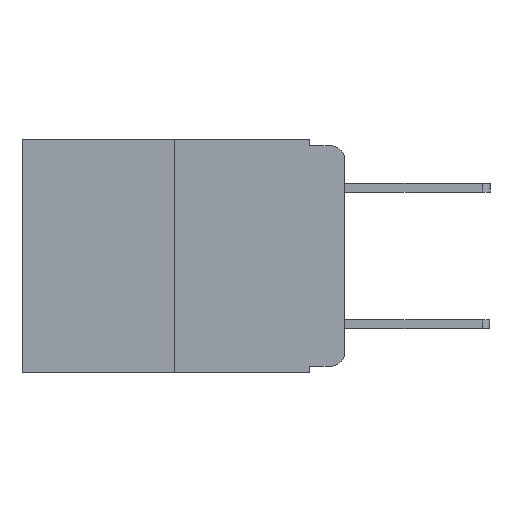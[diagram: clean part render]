
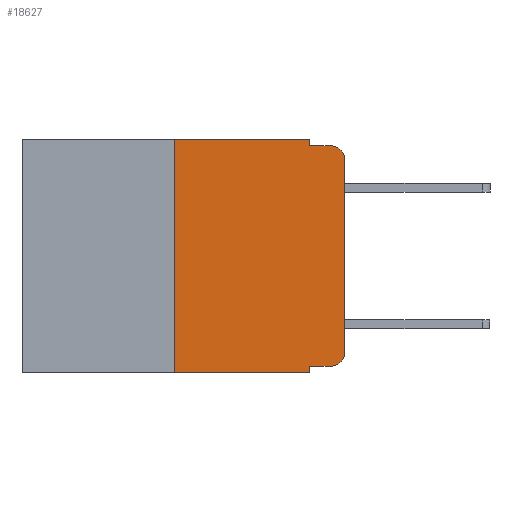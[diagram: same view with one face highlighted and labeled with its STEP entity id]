
A CAD part, left-side view. The second image highlights one B-rep face of the part: STEP entity #18627.
In plain terms, the highlighted planar face has unit normal (-1, 0, 0).
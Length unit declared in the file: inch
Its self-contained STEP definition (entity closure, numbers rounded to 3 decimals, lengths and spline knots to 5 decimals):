
#296 = EDGE_CURVE ( 'NONE', #11384, #21866, #13448, .T. ) ;
#1138 = EDGE_CURVE ( 'NONE', #13614, #17031, #17412, .T. ) ;
#1396 = DIRECTION ( 'NONE',  ( 0., 0., 1. ) ) ;
#1553 = AXIS2_PLACEMENT_3D ( 'NONE', #15737, #6686, #19331 ) ;
#2285 = LINE ( 'NONE', #16118, #21654 ) ;
#2743 = CARTESIAN_POINT ( 'NONE',  ( 0., 0.051, -0.01 ) ) ;
#2952 = LINE ( 'NONE', #21326, #12137 ) ;
#3007 = ORIENTED_EDGE ( 'NONE', *, *, #14702, .T. ) ;
#3211 = CARTESIAN_POINT ( 'NONE',  ( 0., 0.02, -0.313 ) ) ;
#3854 = ORIENTED_EDGE ( 'NONE', *, *, #9864, .T. ) ;
#3961 = LINE ( 'NONE', #22423, #22634 ) ;
#4068 = DIRECTION ( 'NONE',  ( 0., 0., 1. ) ) ;
#4668 = DIRECTION ( 'NONE',  ( 0., 0., -1. ) ) ;
#4932 = EDGE_CURVE ( 'NONE', #19876, #9130, #18356, .T. ) ;
#5097 = VERTEX_POINT ( 'NONE', #12315 ) ;
#5102 = DIRECTION ( 'NONE',  ( 0., 0., -1. ) ) ;
#5242 = ORIENTED_EDGE ( 'NONE', *, *, #1138, .F. ) ;
#6686 = DIRECTION ( 'NONE',  ( 1., 0., 0. ) ) ;
#6777 = VECTOR ( 'NONE', #17900, 39.37008 ) ;
#7019 = ORIENTED_EDGE ( 'NONE', *, *, #12694, .T. ) ;
#7084 = DIRECTION ( 'NONE',  ( 0., 0., -1. ) ) ;
#7363 = LINE ( 'NONE', #19692, #6777 ) ;
#7466 = VERTEX_POINT ( 'NONE', #7899 ) ;
#7638 = VERTEX_POINT ( 'NONE', #2743 ) ;
#7899 = CARTESIAN_POINT ( 'NONE',  ( 0., 0.02, -0.333 ) ) ;
#8380 = ORIENTED_EDGE ( 'NONE', *, *, #12528, .T. ) ;
#8701 = VECTOR ( 'NONE', #21190, 39.37008 ) ;
#8962 = CIRCLE ( 'NONE', #17912, 0.02 ) ;
#9130 = VERTEX_POINT ( 'NONE', #11757 ) ;
#9292 = VECTOR ( 'NONE', #1396, 39.37008 ) ;
#9864 = EDGE_CURVE ( 'NONE', #19876, #7466, #2952, .T. ) ;
#10073 = CIRCLE ( 'NONE', #15921, 0.02 ) ;
#10935 = ORIENTED_EDGE ( 'NONE', *, *, #17503, .F. ) ;
#10971 = CARTESIAN_POINT ( 'NONE',  ( 0., 0.02, -0.03 ) ) ;
#11266 = FACE_OUTER_BOUND ( 'NONE', #13035, .T. ) ;
#11276 = CARTESIAN_POINT ( 'NONE',  ( 0., 0., -0.313 ) ) ;
#11384 = VERTEX_POINT ( 'NONE', #11276 ) ;
#11389 = CARTESIAN_POINT ( 'NONE',  ( 0., 0.25, 0. ) ) ;
#11757 = CARTESIAN_POINT ( 'NONE',  ( 0., 0.051, -0.343 ) ) ;
#11988 = CARTESIAN_POINT ( 'NONE',  ( 0., 0., -0.03 ) ) ;
#12013 = CARTESIAN_POINT ( 'NONE',  ( 0., 0.051, -0.333 ) ) ;
#12137 = VECTOR ( 'NONE', #14176, 39.37008 ) ;
#12315 = CARTESIAN_POINT ( 'NONE',  ( 0., 0.02, -0.01 ) ) ;
#12528 = EDGE_CURVE ( 'NONE', #13614, #9130, #18280, .T. ) ;
#12562 = VECTOR ( 'NONE', #4068, 39.37008 ) ;
#12589 = CARTESIAN_POINT ( 'NONE',  ( 0., 0.25, 0. ) ) ;
#12647 = ORIENTED_EDGE ( 'NONE', *, *, #296, .T. ) ;
#12694 = EDGE_CURVE ( 'NONE', #21866, #5097, #10073, .T. ) ;
#12733 = DIRECTION ( 'NONE',  ( 0., 0., -1. ) ) ;
#13035 = EDGE_LOOP ( 'NONE', ( #12647, #7019, #14394, #19072, #10935, #5242, #8380, #16072, #3854, #3007 ) ) ;
#13448 = LINE ( 'NONE', #17903, #9292 ) ;
#13614 = VERTEX_POINT ( 'NONE', #20679 ) ;
#14104 = VECTOR ( 'NONE', #4668, 39.37008 ) ;
#14176 = DIRECTION ( 'NONE',  ( 0., -1., 0. ) ) ;
#14394 = ORIENTED_EDGE ( 'NONE', *, *, #15150, .F. ) ;
#14702 = EDGE_CURVE ( 'NONE', #7466, #11384, #8962, .T. ) ;
#15150 = EDGE_CURVE ( 'NONE', #7638, #5097, #3961, .T. ) ;
#15601 = CARTESIAN_POINT ( 'NONE',  ( 0., 0.051, 0. ) ) ;
#15737 = CARTESIAN_POINT ( 'NONE',  ( 0., 0.473, 0. ) ) ;
#15921 = AXIS2_PLACEMENT_3D ( 'NONE', #10971, #23434, #12733 ) ;
#16020 = DIRECTION ( 'NONE',  ( -1., 0., 0. ) ) ;
#16072 = ORIENTED_EDGE ( 'NONE', *, *, #4932, .F. ) ;
#16118 = CARTESIAN_POINT ( 'NONE',  ( 0., 0.051, 0. ) ) ;
#17031 = VERTEX_POINT ( 'NONE', #12589 ) ;
#17174 = DIRECTION ( 'NONE',  ( 0., -1., 0. ) ) ;
#17412 = LINE ( 'NONE', #11389, #12562 ) ;
#17503 = EDGE_CURVE ( 'NONE', #17031, #22136, #7363, .T. ) ;
#17900 = DIRECTION ( 'NONE',  ( 0., -1., 0. ) ) ;
#17903 = CARTESIAN_POINT ( 'NONE',  ( 0., 0., 0. ) ) ;
#17912 = AXIS2_PLACEMENT_3D ( 'NONE', #3211, #16020, #5102 ) ;
#18238 = CARTESIAN_POINT ( 'NONE',  ( 0., 0.051, 0. ) ) ;
#18280 = LINE ( 'NONE', #19401, #8701 ) ;
#18356 = LINE ( 'NONE', #15601, #14104 ) ;
#18627 = ADVANCED_FACE ( 'NONE', ( #11266 ), #22770, .F. ) ;
#18768 = EDGE_CURVE ( 'NONE', #22136, #7638, #2285, .T. ) ;
#19072 = ORIENTED_EDGE ( 'NONE', *, *, #18768, .F. ) ;
#19331 = DIRECTION ( 'NONE',  ( 0., 0., -1. ) ) ;
#19401 = CARTESIAN_POINT ( 'NONE',  ( 0., 0.473, -0.343 ) ) ;
#19692 = CARTESIAN_POINT ( 'NONE',  ( 0., 0.473, 0. ) ) ;
#19876 = VERTEX_POINT ( 'NONE', #12013 ) ;
#20679 = CARTESIAN_POINT ( 'NONE',  ( 0., 0.25, -0.343 ) ) ;
#21190 = DIRECTION ( 'NONE',  ( 0., -1., 0. ) ) ;
#21326 = CARTESIAN_POINT ( 'NONE',  ( 0., 0.051, -0.333 ) ) ;
#21654 = VECTOR ( 'NONE', #7084, 39.37008 ) ;
#21866 = VERTEX_POINT ( 'NONE', #11988 ) ;
#22136 = VERTEX_POINT ( 'NONE', #18238 ) ;
#22423 = CARTESIAN_POINT ( 'NONE',  ( 0., 0.051, -0.01 ) ) ;
#22634 = VECTOR ( 'NONE', #17174, 39.37008 ) ;
#22770 = PLANE ( 'NONE',  #1553 ) ;
#23434 = DIRECTION ( 'NONE',  ( -1., 0., 0. ) ) ;
